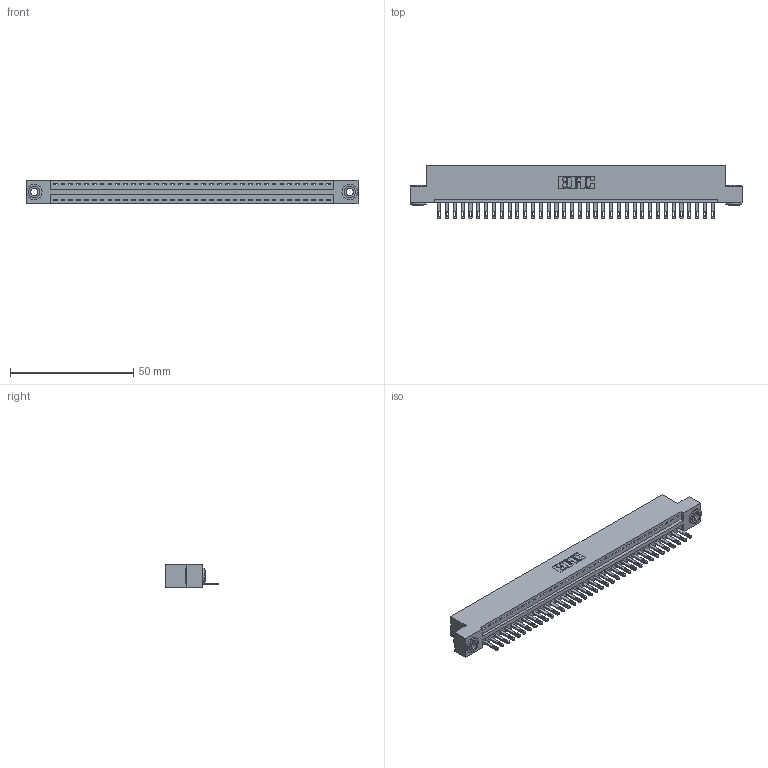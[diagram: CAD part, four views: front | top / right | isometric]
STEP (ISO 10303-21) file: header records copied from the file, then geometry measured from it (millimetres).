
FILE_DESCRIPTION (( 'STEP AP203' ), '1' );
FILE_NAME ('896-036-500-103.STEP', '2021-07-27T20:05:43', ( '' ), ( '' ), 'SwSTEP 2.0', 'SolidWorks 2020', '' );
FILE_SCHEMA (( 'CONFIG_CONTROL_DESIGN' ));
Length unit declared in the file: inch
Products named in the file (4): 345-292-001_345-293-100; 345-250-002_345-250-002-102; 896-036-500-103; 846 Part_Flush Mounting Lugs - 0.156 Dia-TH
Assembly tree (39 placements, depth 2):
  896-036-500-103
    846 Part_Flush Mounting Lugs - 0.156 Dia-TH
    345-292-001_345-293-100  x36
    345-250-002_345-250-002-102  x2
Bounding box: 134.87 x 21.84 x 9.4 mm (x, y, z)
Volume: 12910.8 mm3; surface area: 16375.1 mm2
Topology: 39 solids, 39 shells, 2104 faces, 6453 edges, 4298 vertices
Faces by surface type: plane 1310, cylinder 786, cone 8
Entity records: 23730 total; most frequent: CARTESIAN_POINT 4047, ORIENTED_EDGE 4010, DIRECTION 3611, EDGE_CURVE 2005, LINE 1701, VECTOR 1701, VERTEX_POINT 1334, AXIS2_PLACEMENT_3D 955
